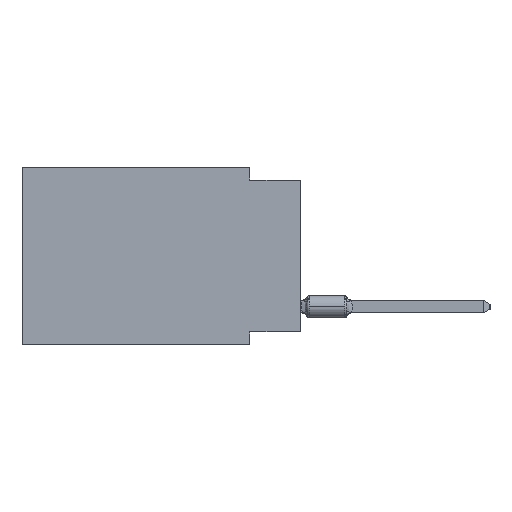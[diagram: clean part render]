
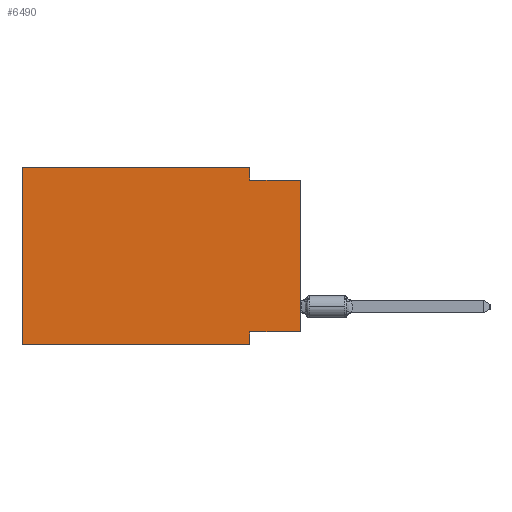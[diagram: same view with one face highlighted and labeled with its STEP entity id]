
A CAD part, left-side view. The second image highlights one B-rep face of the part: STEP entity #6490.
In plain terms, the highlighted planar face has unit normal (-1, 0, 0).
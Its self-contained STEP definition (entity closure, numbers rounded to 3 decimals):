
#697 = EDGE_CURVE ( 'NONE', #19390, #19728, #1826, .T. ) ;
#753 = EDGE_CURVE ( 'NONE', #3893, #13099, #13701, .T. ) ;
#875 = LINE ( 'NONE', #15089, #10776 ) ;
#888 = LINE ( 'NONE', #7199, #17765 ) ;
#1541 = ORIENTED_EDGE ( 'NONE', *, *, #697, .F. ) ;
#1674 = CARTESIAN_POINT ( 'NONE',  ( 0., 13.97, 0. ) ) ;
#1826 = LINE ( 'NONE', #3432, #8815 ) ;
#2732 = CARTESIAN_POINT ( 'NONE',  ( 0., 2.54, -8.255 ) ) ;
#2753 = ORIENTED_EDGE ( 'NONE', *, *, #15978, .F. ) ;
#3228 = VECTOR ( 'NONE', #6673, 1000. ) ;
#3255 = ORIENTED_EDGE ( 'NONE', *, *, #19378, .F. ) ;
#3432 = CARTESIAN_POINT ( 'NONE',  ( 0., 2.54, -8.89 ) ) ;
#3699 = PLANE ( 'NONE',  #16514 ) ;
#3893 = VERTEX_POINT ( 'NONE', #15902 ) ;
#3969 = CARTESIAN_POINT ( 'NONE',  ( 0., 13.97, 0. ) ) ;
#4029 = VECTOR ( 'NONE', #9166, 1000. ) ;
#5957 = CARTESIAN_POINT ( 'NONE',  ( 0., 0., -8.255 ) ) ;
#6066 = EDGE_CURVE ( 'NONE', #17860, #9393, #20877, .T. ) ;
#6490 = ADVANCED_FACE ( 'NONE', ( #11924 ), #3699, .F. ) ;
#6673 = DIRECTION ( 'NONE',  ( 0., -1., 0. ) ) ;
#6924 = CARTESIAN_POINT ( 'NONE',  ( 0., 0., 0. ) ) ;
#7199 = CARTESIAN_POINT ( 'NONE',  ( 0., 2.54, 0. ) ) ;
#7446 = LINE ( 'NONE', #10856, #15048 ) ;
#7545 = DIRECTION ( 'NONE',  ( 0., 1., 0. ) ) ;
#7622 = CARTESIAN_POINT ( 'NONE',  ( 0., 2.54, -8.89 ) ) ;
#7893 = EDGE_CURVE ( 'NONE', #13099, #17186, #875, .T. ) ;
#8572 = ORIENTED_EDGE ( 'NONE', *, *, #11114, .T. ) ;
#8815 = VECTOR ( 'NONE', #16490, 1000. ) ;
#8818 = CARTESIAN_POINT ( 'NONE',  ( 0., 13.97, 0. ) ) ;
#9166 = DIRECTION ( 'NONE',  ( 0., -1., 0. ) ) ;
#9393 = VERTEX_POINT ( 'NONE', #12707 ) ;
#9424 = ORIENTED_EDGE ( 'NONE', *, *, #7893, .F. ) ;
#10668 = CARTESIAN_POINT ( 'NONE',  ( 0., 0., -0.635 ) ) ;
#10776 = VECTOR ( 'NONE', #18427, 1000. ) ;
#10856 = CARTESIAN_POINT ( 'NONE',  ( 0., 0., -8.255 ) ) ;
#11114 = EDGE_CURVE ( 'NONE', #3893, #19728, #20338, .T. ) ;
#11924 = FACE_OUTER_BOUND ( 'NONE', #12095, .T. ) ;
#12095 = EDGE_LOOP ( 'NONE', ( #17407, #2753, #19069, #9424, #20807, #8572, #1541, #3255 ) ) ;
#12707 = CARTESIAN_POINT ( 'NONE',  ( 0., 0., -0.635 ) ) ;
#13099 = VERTEX_POINT ( 'NONE', #1674 ) ;
#13118 = CARTESIAN_POINT ( 'NONE',  ( 0., 2.54, -0.635 ) ) ;
#13409 = CARTESIAN_POINT ( 'NONE',  ( 0., 13.97, -8.89 ) ) ;
#13593 = DIRECTION ( 'NONE',  ( 0., 0., 1. ) ) ;
#13701 = LINE ( 'NONE', #3969, #17375 ) ;
#15048 = VECTOR ( 'NONE', #7545, 1000. ) ;
#15089 = CARTESIAN_POINT ( 'NONE',  ( 0., 13.97, 0. ) ) ;
#15902 = CARTESIAN_POINT ( 'NONE',  ( 0., 13.97, -8.89 ) ) ;
#15978 = EDGE_CURVE ( 'NONE', #19123, #9393, #18822, .T. ) ;
#16490 = DIRECTION ( 'NONE',  ( 0., 0., -1. ) ) ;
#16514 = AXIS2_PLACEMENT_3D ( 'NONE', #8818, #18252, #20169 ) ;
#16983 = EDGE_CURVE ( 'NONE', #17186, #19123, #888, .T. ) ;
#17186 = VERTEX_POINT ( 'NONE', #19168 ) ;
#17366 = DIRECTION ( 'NONE',  ( 0., 0., -1. ) ) ;
#17375 = VECTOR ( 'NONE', #13593, 1000. ) ;
#17407 = ORIENTED_EDGE ( 'NONE', *, *, #6066, .T. ) ;
#17765 = VECTOR ( 'NONE', #17366, 1000. ) ;
#17860 = VERTEX_POINT ( 'NONE', #5957 ) ;
#18252 = DIRECTION ( 'NONE',  ( 1., 0., 0. ) ) ;
#18427 = DIRECTION ( 'NONE',  ( 0., -1., 0. ) ) ;
#18582 = VECTOR ( 'NONE', #19873, 1000. ) ;
#18822 = LINE ( 'NONE', #10668, #4029 ) ;
#19069 = ORIENTED_EDGE ( 'NONE', *, *, #16983, .F. ) ;
#19123 = VERTEX_POINT ( 'NONE', #13118 ) ;
#19168 = CARTESIAN_POINT ( 'NONE',  ( 0., 2.54, 0. ) ) ;
#19378 = EDGE_CURVE ( 'NONE', #17860, #19390, #7446, .T. ) ;
#19390 = VERTEX_POINT ( 'NONE', #2732 ) ;
#19728 = VERTEX_POINT ( 'NONE', #7622 ) ;
#19873 = DIRECTION ( 'NONE',  ( 0., 0., 1. ) ) ;
#20169 = DIRECTION ( 'NONE',  ( 0., 0., -1. ) ) ;
#20338 = LINE ( 'NONE', #13409, #3228 ) ;
#20807 = ORIENTED_EDGE ( 'NONE', *, *, #753, .F. ) ;
#20877 = LINE ( 'NONE', #6924, #18582 ) ;
